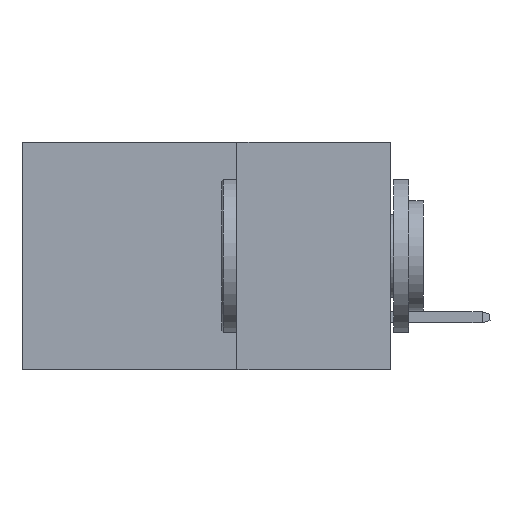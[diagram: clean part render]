
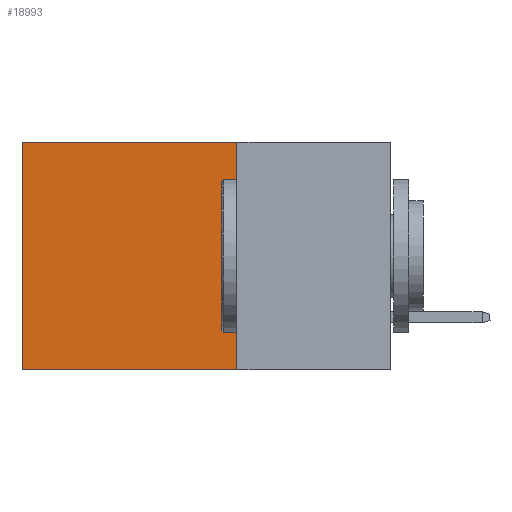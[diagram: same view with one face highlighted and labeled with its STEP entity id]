
A CAD part, left-side view. The second image highlights one B-rep face of the part: STEP entity #18993.
In plain terms, the highlighted planar face has unit normal (-1, 0, 0).
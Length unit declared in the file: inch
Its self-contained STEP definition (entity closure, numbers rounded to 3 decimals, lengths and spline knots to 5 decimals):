
#133 = LINE ( 'NONE', #30998, #19328 ) ;
#428 = CARTESIAN_POINT ( 'NONE',  ( 0.2875, 0.6, -0.37 ) ) ;
#1085 = ORIENTED_EDGE ( 'NONE', *, *, #30979, .T. ) ;
#2398 = ORIENTED_EDGE ( 'NONE', *, *, #11295, .F. ) ;
#3578 = CARTESIAN_POINT ( 'NONE',  ( 0.2875, 0.25, -0.37 ) ) ;
#3654 = DIRECTION ( 'NONE',  ( 0., 1., 0. ) ) ;
#3724 = PLANE ( 'NONE',  #16958 ) ;
#4304 = VERTEX_POINT ( 'NONE', #12238 ) ;
#5467 = VECTOR ( 'NONE', #17353, 39.37008 ) ;
#6087 = LINE ( 'NONE', #17116, #11202 ) ;
#6268 = LINE ( 'NONE', #12228, #5467 ) ;
#8819 = DIRECTION ( 'NONE',  ( 1., 0., 0. ) ) ;
#9689 = VERTEX_POINT ( 'NONE', #27603 ) ;
#11202 = VECTOR ( 'NONE', #19553, 39.37008 ) ;
#11225 = ORIENTED_EDGE ( 'NONE', *, *, #18287, .T. ) ;
#11295 = EDGE_CURVE ( 'NONE', #9689, #16332, #6268, .T. ) ;
#12228 = CARTESIAN_POINT ( 'NONE',  ( 0.2875, 0.25, 0. ) ) ;
#12238 = CARTESIAN_POINT ( 'NONE',  ( 0.2875, 0.6, 0. ) ) ;
#16332 = VERTEX_POINT ( 'NONE', #3578 ) ;
#16958 = AXIS2_PLACEMENT_3D ( 'NONE', #26067, #8819, #26188 ) ;
#17116 = CARTESIAN_POINT ( 'NONE',  ( 0.2875, 0.25, -0.37 ) ) ;
#17282 = EDGE_CURVE ( 'NONE', #16332, #18773, #6087, .T. ) ;
#17353 = DIRECTION ( 'NONE',  ( 0., 0., -1. ) ) ;
#18287 = EDGE_CURVE ( 'NONE', #9689, #4304, #133, .T. ) ;
#18773 = VERTEX_POINT ( 'NONE', #428 ) ;
#18993 = ADVANCED_FACE ( 'NONE', ( #30527 ), #3724, .F. ) ;
#19328 = VECTOR ( 'NONE', #3654, 39.37008 ) ;
#19553 = DIRECTION ( 'NONE',  ( 0., 1., 0. ) ) ;
#23450 = VECTOR ( 'NONE', #25155, 39.37008 ) ;
#24474 = EDGE_LOOP ( 'NONE', ( #1085, #29063, #2398, #11225 ) ) ;
#25155 = DIRECTION ( 'NONE',  ( 0., 0., -1. ) ) ;
#26067 = CARTESIAN_POINT ( 'NONE',  ( 0.2875, 0.25, 0. ) ) ;
#26188 = DIRECTION ( 'NONE',  ( 0., 0., -1. ) ) ;
#27603 = CARTESIAN_POINT ( 'NONE',  ( 0.2875, 0.25, 0. ) ) ;
#27675 = CARTESIAN_POINT ( 'NONE',  ( 0.2875, 0.6, 0. ) ) ;
#29063 = ORIENTED_EDGE ( 'NONE', *, *, #17282, .F. ) ;
#30049 = LINE ( 'NONE', #27675, #23450 ) ;
#30527 = FACE_OUTER_BOUND ( 'NONE', #24474, .T. ) ;
#30979 = EDGE_CURVE ( 'NONE', #4304, #18773, #30049, .T. ) ;
#30998 = CARTESIAN_POINT ( 'NONE',  ( 0.2875, 0.25, 0. ) ) ;
